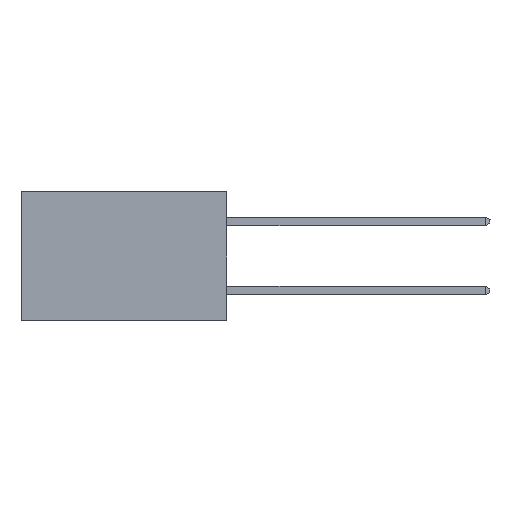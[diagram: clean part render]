
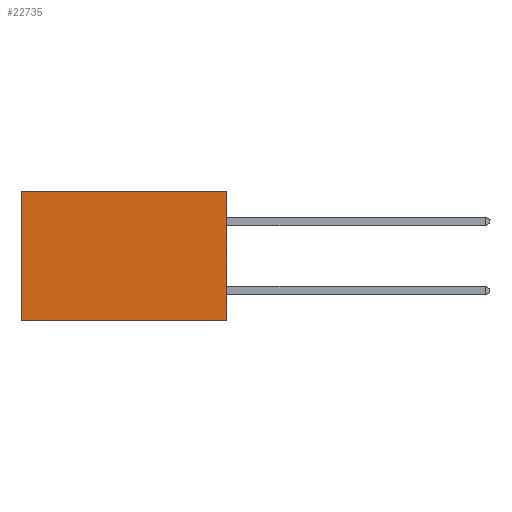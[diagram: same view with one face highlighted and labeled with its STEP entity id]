
A CAD part, left-side view. The second image highlights one B-rep face of the part: STEP entity #22735.
In plain terms, the highlighted planar face has unit normal (-1, 0, 0).
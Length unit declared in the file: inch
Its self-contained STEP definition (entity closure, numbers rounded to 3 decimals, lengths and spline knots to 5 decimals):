
#776 = EDGE_CURVE ( 'NONE', #3280, #16690, #19467, .T. ) ;
#3280 = VERTEX_POINT ( 'NONE', #20993 ) ;
#3529 = CARTESIAN_POINT ( 'NONE',  ( 0.277, 0., -0.37 ) ) ;
#3594 = ORIENTED_EDGE ( 'NONE', *, *, #4507, .F. ) ;
#4507 = EDGE_CURVE ( 'NONE', #3280, #8978, #15402, .T. ) ;
#4633 = CARTESIAN_POINT ( 'NONE',  ( 0.277, 0., -0.37 ) ) ;
#4792 = VECTOR ( 'NONE', #21109, 39.37008 ) ;
#5600 = DIRECTION ( 'NONE',  ( 0., 1., 0. ) ) ;
#6800 = DIRECTION ( 'NONE',  ( 0., 1., 0. ) ) ;
#7767 = PLANE ( 'NONE',  #15797 ) ;
#8740 = CARTESIAN_POINT ( 'NONE',  ( 0.277, 0.59, 0. ) ) ;
#8978 = VERTEX_POINT ( 'NONE', #18593 ) ;
#9704 = LINE ( 'NONE', #12771, #14930 ) ;
#10712 = DIRECTION ( 'NONE',  ( 0., 0., -1. ) ) ;
#11125 = EDGE_CURVE ( 'NONE', #8978, #12871, #12798, .T. ) ;
#12771 = CARTESIAN_POINT ( 'NONE',  ( 0.277, 0.59, -0.37 ) ) ;
#12798 = LINE ( 'NONE', #3529, #22400 ) ;
#12871 = VERTEX_POINT ( 'NONE', #24240 ) ;
#12887 = EDGE_CURVE ( 'NONE', #16690, #12871, #9704, .T. ) ;
#13484 = EDGE_LOOP ( 'NONE', ( #13626, #23800, #3594, #24395 ) ) ;
#13626 = ORIENTED_EDGE ( 'NONE', *, *, #12887, .T. ) ;
#14930 = VECTOR ( 'NONE', #16683, 39.37008 ) ;
#15402 = LINE ( 'NONE', #20456, #4792 ) ;
#15797 = AXIS2_PLACEMENT_3D ( 'NONE', #4633, #22279, #10712 ) ;
#16683 = DIRECTION ( 'NONE',  ( 0., 0., -1. ) ) ;
#16690 = VERTEX_POINT ( 'NONE', #8740 ) ;
#18593 = CARTESIAN_POINT ( 'NONE',  ( 0.277, 0., -0.37 ) ) ;
#19467 = LINE ( 'NONE', #24274, #25095 ) ;
#20456 = CARTESIAN_POINT ( 'NONE',  ( 0.277, 0., -0.37 ) ) ;
#20993 = CARTESIAN_POINT ( 'NONE',  ( 0.277, 0., 0. ) ) ;
#21109 = DIRECTION ( 'NONE',  ( 0., 0., -1. ) ) ;
#22279 = DIRECTION ( 'NONE',  ( 1., 0., 0. ) ) ;
#22400 = VECTOR ( 'NONE', #5600, 39.37008 ) ;
#22735 = ADVANCED_FACE ( 'NONE', ( #22847 ), #7767, .F. ) ;
#22847 = FACE_OUTER_BOUND ( 'NONE', #13484, .T. ) ;
#23800 = ORIENTED_EDGE ( 'NONE', *, *, #11125, .F. ) ;
#24240 = CARTESIAN_POINT ( 'NONE',  ( 0.277, 0.59, -0.37 ) ) ;
#24274 = CARTESIAN_POINT ( 'NONE',  ( 0.277, 0., 0. ) ) ;
#24395 = ORIENTED_EDGE ( 'NONE', *, *, #776, .T. ) ;
#25095 = VECTOR ( 'NONE', #6800, 39.37008 ) ;
